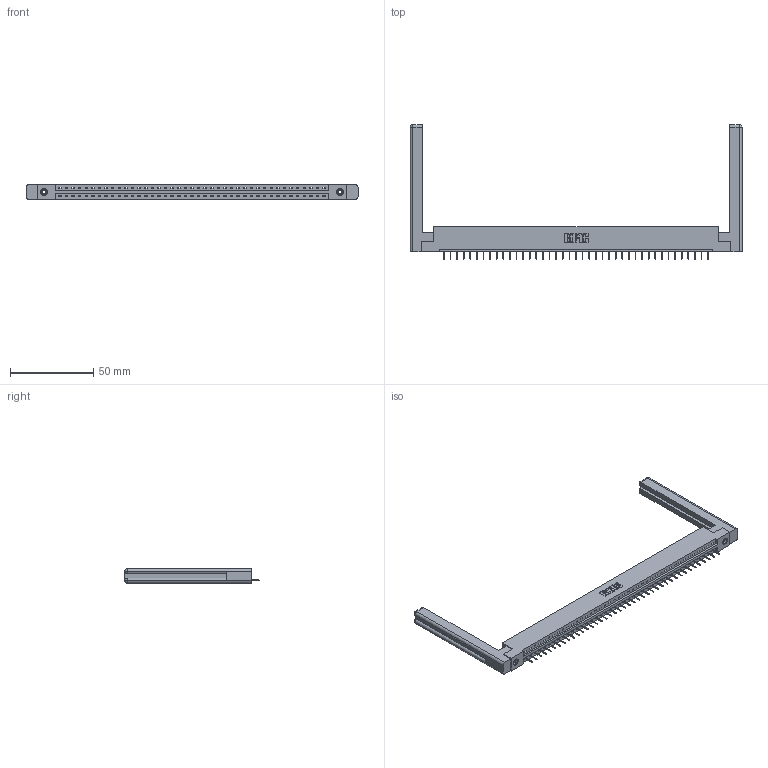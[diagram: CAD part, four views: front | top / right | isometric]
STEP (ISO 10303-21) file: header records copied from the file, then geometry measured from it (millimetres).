
FILE_DESCRIPTION (( 'STEP AP203' ), '1' );
FILE_NAME ('387-041-524-158.STEP', '2019-10-04T19:41:25', ( '' ), ( '' ), 'SwSTEP 2.0', 'SolidWorks 2016', '' );
FILE_SCHEMA (( 'CONFIG_CONTROL_DESIGN' ));
Length unit declared in the file: inch
Products named in the file (5): 345-292-001_345-293-124; 307-220-058; 345-250-001_345-250-001-102; 337 Part_Flush Mounting Lugs - 0.156 Dia-TI; 387-041-524-158
Assembly tree (46 placements, depth 2):
  387-041-524-158
    337 Part_Flush Mounting Lugs - 0.156 Dia-TI
    345-292-001_345-293-124  x41
    345-250-001_345-250-001-102  x2
    307-220-058  x2
Bounding box: 199.09 x 80.78 x 9.4 mm (x, y, z)
Volume: 27679.2 mm3; surface area: 25839.3 mm2
Topology: 46 solids, 46 shells, 2962 faces, 8537 edges, 5514 vertices
Faces by surface type: plane 2286, cylinder 652, cone 12, torus 12
Entity records: 33314 total; most frequent: CARTESIAN_POINT 5800, ORIENTED_EDGE 5716, DIRECTION 4904, EDGE_CURVE 2858, LINE 2686, VECTOR 2686, VERTEX_POINT 1894, AXIS2_PLACEMENT_3D 1109
